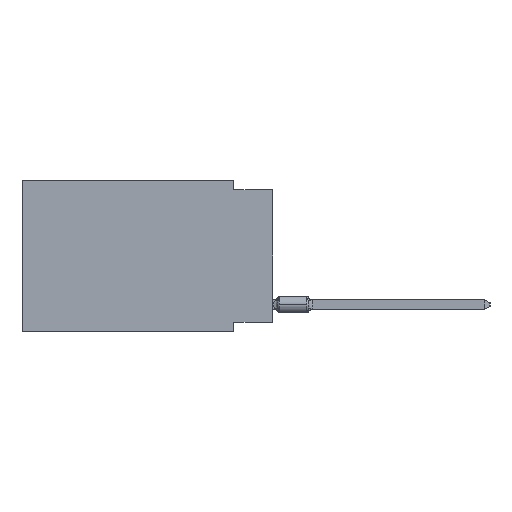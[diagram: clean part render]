
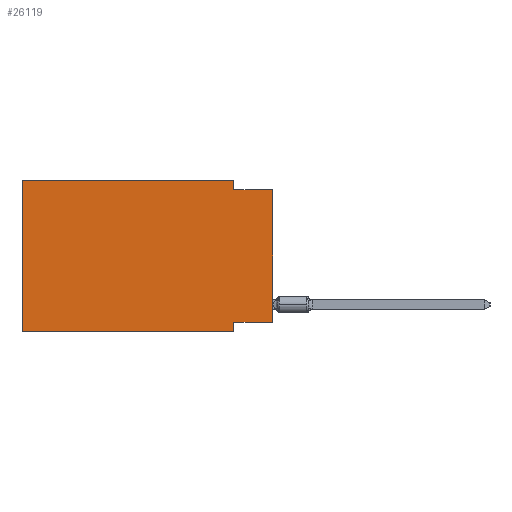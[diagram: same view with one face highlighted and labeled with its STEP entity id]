
A CAD part, left-side view. The second image highlights one B-rep face of the part: STEP entity #26119.
In plain terms, the highlighted planar face has unit normal (-1, 0, 0).
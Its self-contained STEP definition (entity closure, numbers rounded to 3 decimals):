
#574 = VERTEX_POINT ( 'NONE', #25078 ) ;
#1147 = VERTEX_POINT ( 'NONE', #12041 ) ;
#1150 = LINE ( 'NONE', #12018, #6965 ) ;
#1357 = CARTESIAN_POINT ( 'NONE',  ( 0., 0., -0.635 ) ) ;
#2665 = LINE ( 'NONE', #2838, #27872 ) ;
#2832 = CARTESIAN_POINT ( 'NONE',  ( 0., 16.383, 0. ) ) ;
#2838 = CARTESIAN_POINT ( 'NONE',  ( 0., 2.54, 0. ) ) ;
#2875 = AXIS2_PLACEMENT_3D ( 'NONE', #5907, #19610, #5244 ) ;
#3301 = CARTESIAN_POINT ( 'NONE',  ( 0., 0., -9.271 ) ) ;
#4291 = LINE ( 'NONE', #5252, #17869 ) ;
#5244 = DIRECTION ( 'NONE',  ( 0., 0., -1. ) ) ;
#5252 = CARTESIAN_POINT ( 'NONE',  ( 0., 16.383, -9.906 ) ) ;
#5907 = CARTESIAN_POINT ( 'NONE',  ( 0., 16.383, 0. ) ) ;
#6831 = CARTESIAN_POINT ( 'NONE',  ( 0., 2.54, -9.906 ) ) ;
#6965 = VECTOR ( 'NONE', #11849, 1000. ) ;
#8054 = DIRECTION ( 'NONE',  ( 0., -1., 0. ) ) ;
#8067 = VECTOR ( 'NONE', #25523, 1000. ) ;
#8334 = ORIENTED_EDGE ( 'NONE', *, *, #18395, .F. ) ;
#8639 = EDGE_CURVE ( 'NONE', #34410, #574, #11485, .T. ) ;
#8719 = EDGE_CURVE ( 'NONE', #11057, #14155, #1150, .T. ) ;
#10530 = EDGE_CURVE ( 'NONE', #20998, #1147, #4291, .T. ) ;
#11057 = VERTEX_POINT ( 'NONE', #3301 ) ;
#11444 = CARTESIAN_POINT ( 'NONE',  ( 0., 0., 0. ) ) ;
#11485 = LINE ( 'NONE', #17630, #8067 ) ;
#11713 = FACE_OUTER_BOUND ( 'NONE', #21680, .T. ) ;
#11849 = DIRECTION ( 'NONE',  ( 0., 1., 0. ) ) ;
#11979 = LINE ( 'NONE', #11444, #27883 ) ;
#12018 = CARTESIAN_POINT ( 'NONE',  ( 0., 0., -9.271 ) ) ;
#12041 = CARTESIAN_POINT ( 'NONE',  ( 0., 2.54, -9.906 ) ) ;
#12365 = EDGE_CURVE ( 'NONE', #574, #17408, #2665, .T. ) ;
#14155 = VERTEX_POINT ( 'NONE', #18929 ) ;
#14257 = DIRECTION ( 'NONE',  ( 0., 0., -1. ) ) ;
#15496 = VERTEX_POINT ( 'NONE', #1357 ) ;
#15672 = CARTESIAN_POINT ( 'NONE',  ( 0., 16.383, 0. ) ) ;
#16355 = LINE ( 'NONE', #15672, #18271 ) ;
#17385 = ORIENTED_EDGE ( 'NONE', *, *, #8639, .F. ) ;
#17408 = VERTEX_POINT ( 'NONE', #26443 ) ;
#17630 = CARTESIAN_POINT ( 'NONE',  ( 0., 16.383, 0. ) ) ;
#17869 = VECTOR ( 'NONE', #8054, 1000. ) ;
#18271 = VECTOR ( 'NONE', #27038, 1000. ) ;
#18395 = EDGE_CURVE ( 'NONE', #20998, #34410, #16355, .T. ) ;
#18625 = DIRECTION ( 'NONE',  ( 0., 0., -1. ) ) ;
#18922 = CARTESIAN_POINT ( 'NONE',  ( 0., 0., -0.635 ) ) ;
#18929 = CARTESIAN_POINT ( 'NONE',  ( 0., 2.54, -9.271 ) ) ;
#19210 = EDGE_CURVE ( 'NONE', #14155, #1147, #31037, .T. ) ;
#19229 = ORIENTED_EDGE ( 'NONE', *, *, #19210, .F. ) ;
#19425 = PLANE ( 'NONE',  #2875 ) ;
#19610 = DIRECTION ( 'NONE',  ( 1., 0., 0. ) ) ;
#20908 = EDGE_CURVE ( 'NONE', #17408, #15496, #26634, .T. ) ;
#20998 = VERTEX_POINT ( 'NONE', #31274 ) ;
#21680 = EDGE_LOOP ( 'NONE', ( #28824, #29273, #21890, #17385, #8334, #33900, #19229, #30642 ) ) ;
#21890 = ORIENTED_EDGE ( 'NONE', *, *, #12365, .F. ) ;
#22688 = DIRECTION ( 'NONE',  ( 0., 0., 1. ) ) ;
#23267 = VECTOR ( 'NONE', #14257, 1000. ) ;
#23839 = DIRECTION ( 'NONE',  ( 0., -1., 0. ) ) ;
#25078 = CARTESIAN_POINT ( 'NONE',  ( 0., 2.54, 0. ) ) ;
#25523 = DIRECTION ( 'NONE',  ( 0., -1., 0. ) ) ;
#26119 = ADVANCED_FACE ( 'NONE', ( #11713 ), #19425, .F. ) ;
#26121 = VECTOR ( 'NONE', #23839, 1000. ) ;
#26443 = CARTESIAN_POINT ( 'NONE',  ( 0., 2.54, -0.635 ) ) ;
#26634 = LINE ( 'NONE', #18922, #26121 ) ;
#27038 = DIRECTION ( 'NONE',  ( 0., 0., 1. ) ) ;
#27652 = EDGE_CURVE ( 'NONE', #11057, #15496, #11979, .T. ) ;
#27872 = VECTOR ( 'NONE', #18625, 1000. ) ;
#27883 = VECTOR ( 'NONE', #22688, 1000. ) ;
#28824 = ORIENTED_EDGE ( 'NONE', *, *, #27652, .T. ) ;
#29273 = ORIENTED_EDGE ( 'NONE', *, *, #20908, .F. ) ;
#30642 = ORIENTED_EDGE ( 'NONE', *, *, #8719, .F. ) ;
#31037 = LINE ( 'NONE', #6831, #23267 ) ;
#31274 = CARTESIAN_POINT ( 'NONE',  ( 0., 16.383, -9.906 ) ) ;
#33900 = ORIENTED_EDGE ( 'NONE', *, *, #10530, .T. ) ;
#34410 = VERTEX_POINT ( 'NONE', #2832 ) ;
